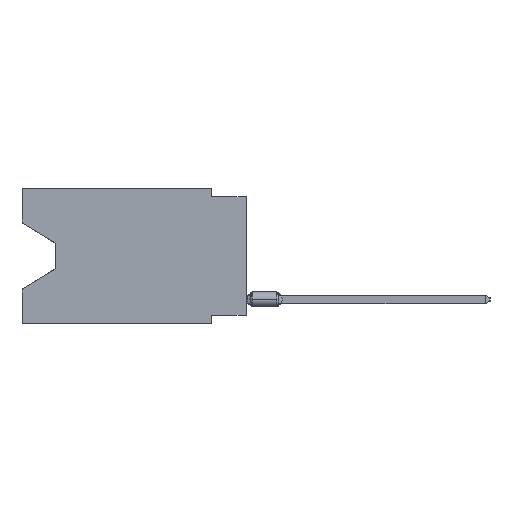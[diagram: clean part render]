
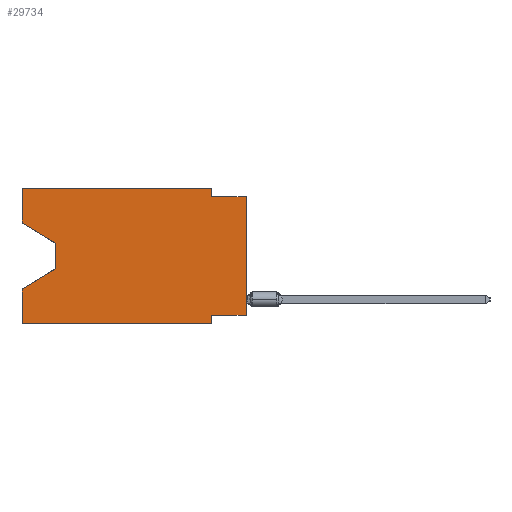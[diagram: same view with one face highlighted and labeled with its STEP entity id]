
A CAD part, left-side view. The second image highlights one B-rep face of the part: STEP entity #29734.
In plain terms, the highlighted planar face has unit normal (-1, 0, 0).
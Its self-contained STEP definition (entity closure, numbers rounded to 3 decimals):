
#338 = CARTESIAN_POINT ( 'NONE',  ( 0., 13.97, -4.013 ) ) ;
#583 = ORIENTED_EDGE ( 'NONE', *, *, #27897, .T. ) ;
#623 = DIRECTION ( 'NONE',  ( 0., 0., 1. ) ) ;
#781 = CARTESIAN_POINT ( 'NONE',  ( 0., 16.383, -2.546 ) ) ;
#1699 = EDGE_CURVE ( 'NONE', #8991, #30234, #21394, .T. ) ;
#2389 = VECTOR ( 'NONE', #623, 1000. ) ;
#2718 = CARTESIAN_POINT ( 'NONE',  ( 0., 2.54, -9.271 ) ) ;
#2804 = CARTESIAN_POINT ( 'NONE',  ( 0., 16.383, -9.906 ) ) ;
#2808 = ORIENTED_EDGE ( 'NONE', *, *, #32600, .T. ) ;
#2864 = CARTESIAN_POINT ( 'NONE',  ( 0., 2.54, -9.906 ) ) ;
#3372 = VECTOR ( 'NONE', #23617, 1000. ) ;
#3726 = DIRECTION ( 'NONE',  ( 0., 0., -1. ) ) ;
#4132 = LINE ( 'NONE', #26420, #26504 ) ;
#4314 = LINE ( 'NONE', #26262, #3372 ) ;
#4683 = CARTESIAN_POINT ( 'NONE',  ( 0., 13.97, -5.893 ) ) ;
#4897 = EDGE_CURVE ( 'NONE', #20292, #7781, #28277, .T. ) ;
#5340 = ORIENTED_EDGE ( 'NONE', *, *, #4897, .F. ) ;
#5406 = EDGE_CURVE ( 'NONE', #28076, #12269, #26291, .T. ) ;
#6078 = CARTESIAN_POINT ( 'NONE',  ( 0., 0., -9.271 ) ) ;
#6958 = LINE ( 'NONE', #4683, #34485 ) ;
#6966 = ORIENTED_EDGE ( 'NONE', *, *, #33421, .F. ) ;
#7141 = CARTESIAN_POINT ( 'NONE',  ( 0., 2.54, 0. ) ) ;
#7288 = EDGE_CURVE ( 'NONE', #12269, #28695, #4314, .T. ) ;
#7361 = VERTEX_POINT ( 'NONE', #2864 ) ;
#7472 = DIRECTION ( 'NONE',  ( 0., -0.855, -0.519 ) ) ;
#7781 = VERTEX_POINT ( 'NONE', #21912 ) ;
#8106 = DIRECTION ( 'NONE',  ( 0., 0., -1. ) ) ;
#8109 = AXIS2_PLACEMENT_3D ( 'NONE', #8451, #8803, #3726 ) ;
#8451 = CARTESIAN_POINT ( 'NONE',  ( 0., 16.383, 0. ) ) ;
#8803 = DIRECTION ( 'NONE',  ( 1., 0., 0. ) ) ;
#8991 = VERTEX_POINT ( 'NONE', #15584 ) ;
#10014 = VERTEX_POINT ( 'NONE', #32942 ) ;
#10458 = VECTOR ( 'NONE', #10951, 1000. ) ;
#10865 = CARTESIAN_POINT ( 'NONE',  ( 0., 2.54, -0.635 ) ) ;
#10951 = DIRECTION ( 'NONE',  ( 0., 0., 1. ) ) ;
#11010 = CARTESIAN_POINT ( 'NONE',  ( 0., 16.383, 0. ) ) ;
#11026 = DIRECTION ( 'NONE',  ( 0., 0., -1. ) ) ;
#11084 = FACE_OUTER_BOUND ( 'NONE', #15878, .T. ) ;
#11441 = EDGE_CURVE ( 'NONE', #30171, #7361, #4132, .T. ) ;
#12215 = DIRECTION ( 'NONE',  ( 0., 0.855, -0.519 ) ) ;
#12269 = VERTEX_POINT ( 'NONE', #11010 ) ;
#12340 = ORIENTED_EDGE ( 'NONE', *, *, #5406, .F. ) ;
#12396 = ORIENTED_EDGE ( 'NONE', *, *, #30831, .F. ) ;
#14310 = EDGE_CURVE ( 'NONE', #27238, #7361, #23596, .T. ) ;
#14565 = ORIENTED_EDGE ( 'NONE', *, *, #11441, .T. ) ;
#15584 = CARTESIAN_POINT ( 'NONE',  ( 0., 13.97, -4.013 ) ) ;
#15812 = CARTESIAN_POINT ( 'NONE',  ( 0., 0., -9.271 ) ) ;
#15878 = EDGE_LOOP ( 'NONE', ( #20399, #17429, #583, #34284, #14565, #18373, #6966, #2808, #5340, #12396, #22958, #12340 ) ) ;
#16694 = VERTEX_POINT ( 'NONE', #15812 ) ;
#17128 = LINE ( 'NONE', #24675, #2389 ) ;
#17429 = ORIENTED_EDGE ( 'NONE', *, *, #1699, .T. ) ;
#17736 = CARTESIAN_POINT ( 'NONE',  ( 0., 13.97, -5.893 ) ) ;
#17861 = DIRECTION ( 'NONE',  ( 0., 0., -1. ) ) ;
#18373 = ORIENTED_EDGE ( 'NONE', *, *, #14310, .F. ) ;
#20028 = CARTESIAN_POINT ( 'NONE',  ( 0., 2.54, 0. ) ) ;
#20171 = CARTESIAN_POINT ( 'NONE',  ( 0., 0., -0.635 ) ) ;
#20292 = VERTEX_POINT ( 'NONE', #10865 ) ;
#20399 = ORIENTED_EDGE ( 'NONE', *, *, #32503, .T. ) ;
#20491 = LINE ( 'NONE', #7141, #22500 ) ;
#21178 = VECTOR ( 'NONE', #11026, 1000. ) ;
#21394 = LINE ( 'NONE', #338, #21178 ) ;
#21631 = CARTESIAN_POINT ( 'NONE',  ( 0., 16.383, 0. ) ) ;
#21809 = DIRECTION ( 'NONE',  ( 0., 0., 1. ) ) ;
#21812 = VECTOR ( 'NONE', #30906, 1000. ) ;
#21912 = CARTESIAN_POINT ( 'NONE',  ( 0., 0., -0.635 ) ) ;
#22351 = LINE ( 'NONE', #25002, #10458 ) ;
#22404 = LINE ( 'NONE', #6078, #31269 ) ;
#22500 = VECTOR ( 'NONE', #17861, 1000. ) ;
#22958 = ORIENTED_EDGE ( 'NONE', *, *, #7288, .F. ) ;
#23596 = LINE ( 'NONE', #29554, #31669 ) ;
#23617 = DIRECTION ( 'NONE',  ( 0., -1., 0. ) ) ;
#24076 = VECTOR ( 'NONE', #21809, 1000. ) ;
#24303 = EDGE_CURVE ( 'NONE', #30171, #10014, #17128, .T. ) ;
#24675 = CARTESIAN_POINT ( 'NONE',  ( 0., 16.383, 0. ) ) ;
#25002 = CARTESIAN_POINT ( 'NONE',  ( 0., 0., 0. ) ) ;
#25619 = VECTOR ( 'NONE', #7472, 1000. ) ;
#26262 = CARTESIAN_POINT ( 'NONE',  ( 0., 16.383, 0. ) ) ;
#26291 = LINE ( 'NONE', #21631, #24076 ) ;
#26420 = CARTESIAN_POINT ( 'NONE',  ( 0., 16.383, -9.906 ) ) ;
#26504 = VECTOR ( 'NONE', #31873, 1000. ) ;
#27238 = VERTEX_POINT ( 'NONE', #2718 ) ;
#27266 = PLANE ( 'NONE',  #8109 ) ;
#27897 = EDGE_CURVE ( 'NONE', #30234, #10014, #6958, .T. ) ;
#28076 = VERTEX_POINT ( 'NONE', #781 ) ;
#28277 = LINE ( 'NONE', #20171, #21812 ) ;
#28695 = VERTEX_POINT ( 'NONE', #20028 ) ;
#29554 = CARTESIAN_POINT ( 'NONE',  ( 0., 2.54, -9.906 ) ) ;
#29734 = ADVANCED_FACE ( 'NONE', ( #11084 ), #27266, .F. ) ;
#30152 = DIRECTION ( 'NONE',  ( 0., 1., 0. ) ) ;
#30171 = VERTEX_POINT ( 'NONE', #2804 ) ;
#30234 = VERTEX_POINT ( 'NONE', #17736 ) ;
#30831 = EDGE_CURVE ( 'NONE', #28695, #20292, #20491, .T. ) ;
#30906 = DIRECTION ( 'NONE',  ( 0., -1., 0. ) ) ;
#31269 = VECTOR ( 'NONE', #30152, 1000. ) ;
#31669 = VECTOR ( 'NONE', #8106, 1000. ) ;
#31873 = DIRECTION ( 'NONE',  ( 0., -1., 0. ) ) ;
#32227 = LINE ( 'NONE', #34191, #25619 ) ;
#32503 = EDGE_CURVE ( 'NONE', #28076, #8991, #32227, .T. ) ;
#32600 = EDGE_CURVE ( 'NONE', #16694, #7781, #22351, .T. ) ;
#32942 = CARTESIAN_POINT ( 'NONE',  ( 0., 16.383, -7.36 ) ) ;
#33421 = EDGE_CURVE ( 'NONE', #16694, #27238, #22404, .T. ) ;
#34191 = CARTESIAN_POINT ( 'NONE',  ( 0., 16.383, -2.546 ) ) ;
#34284 = ORIENTED_EDGE ( 'NONE', *, *, #24303, .F. ) ;
#34485 = VECTOR ( 'NONE', #12215, 1000. ) ;
